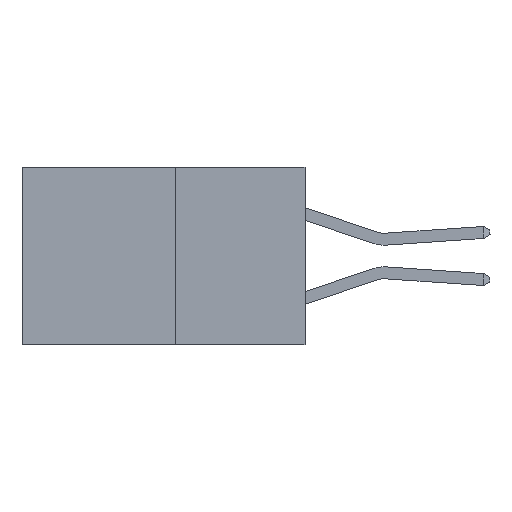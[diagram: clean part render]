
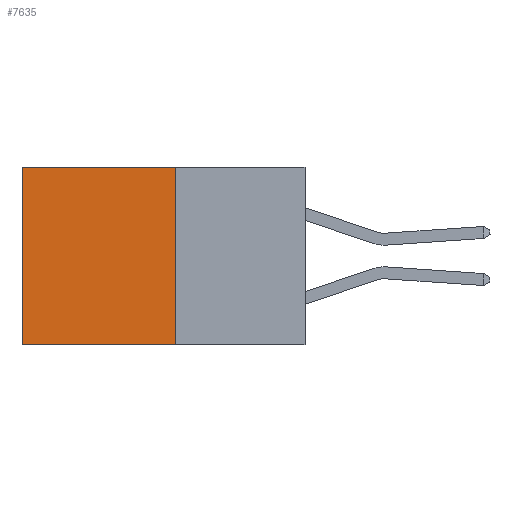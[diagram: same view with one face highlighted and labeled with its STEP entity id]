
A CAD part, left-side view. The second image highlights one B-rep face of the part: STEP entity #7635.
In plain terms, the highlighted planar face has unit normal (-1, 0, 0).
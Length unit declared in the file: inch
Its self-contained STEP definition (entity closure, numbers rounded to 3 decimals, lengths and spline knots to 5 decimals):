
#502 = VECTOR ( 'NONE', #4744, 39.37008 ) ;
#523 = LINE ( 'NONE', #7205, #9008 ) ;
#785 = VECTOR ( 'NONE', #6445, 39.37008 ) ;
#929 = VECTOR ( 'NONE', #1100, 39.37008 ) ;
#1100 = DIRECTION ( 'NONE',  ( 0., 1., 0. ) ) ;
#2003 = EDGE_CURVE ( 'NONE', #2526, #7142, #4891, .T. ) ;
#2526 = VERTEX_POINT ( 'NONE', #4250 ) ;
#2650 = LINE ( 'NONE', #2837, #502 ) ;
#2782 = VERTEX_POINT ( 'NONE', #6584 ) ;
#2837 = CARTESIAN_POINT ( 'NONE',  ( 0.277, 0.27, -0.37 ) ) ;
#4250 = CARTESIAN_POINT ( 'NONE',  ( 0.277, 0.27, 0. ) ) ;
#4744 = DIRECTION ( 'NONE',  ( 0., 1., 0. ) ) ;
#4891 = LINE ( 'NONE', #8728, #785 ) ;
#5030 = CARTESIAN_POINT ( 'NONE',  ( 0.277, 0.59, -0.37 ) ) ;
#5105 = EDGE_CURVE ( 'NONE', #2526, #2782, #5284, .T. ) ;
#5284 = LINE ( 'NONE', #9351, #929 ) ;
#5449 = ORIENTED_EDGE ( 'NONE', *, *, #6275, .T. ) ;
#6275 = EDGE_CURVE ( 'NONE', #2782, #9321, #523, .T. ) ;
#6445 = DIRECTION ( 'NONE',  ( 0., 0., -1. ) ) ;
#6584 = CARTESIAN_POINT ( 'NONE',  ( 0.277, 0.59, 0. ) ) ;
#6620 = EDGE_LOOP ( 'NONE', ( #5449, #6915, #9534, #7563 ) ) ;
#6915 = ORIENTED_EDGE ( 'NONE', *, *, #7897, .F. ) ;
#7142 = VERTEX_POINT ( 'NONE', #7643 ) ;
#7205 = CARTESIAN_POINT ( 'NONE',  ( 0.277, 0.59, -0.37 ) ) ;
#7265 = DIRECTION ( 'NONE',  ( 0., 0., -1. ) ) ;
#7563 = ORIENTED_EDGE ( 'NONE', *, *, #5105, .T. ) ;
#7635 = ADVANCED_FACE ( 'NONE', ( #9346 ), #8468, .F. ) ;
#7643 = CARTESIAN_POINT ( 'NONE',  ( 0.277, 0.27, -0.37 ) ) ;
#7709 = DIRECTION ( 'NONE',  ( 0., 0., -1. ) ) ;
#7897 = EDGE_CURVE ( 'NONE', #7142, #9321, #2650, .T. ) ;
#8468 = PLANE ( 'NONE',  #8765 ) ;
#8652 = CARTESIAN_POINT ( 'NONE',  ( 0.277, 0.27, -0.37 ) ) ;
#8728 = CARTESIAN_POINT ( 'NONE',  ( 0.277, 0.27, -0.37 ) ) ;
#8765 = AXIS2_PLACEMENT_3D ( 'NONE', #8652, #10031, #7709 ) ;
#9008 = VECTOR ( 'NONE', #7265, 39.37008 ) ;
#9321 = VERTEX_POINT ( 'NONE', #5030 ) ;
#9346 = FACE_OUTER_BOUND ( 'NONE', #6620, .T. ) ;
#9351 = CARTESIAN_POINT ( 'NONE',  ( 0.277, 0.27, 0. ) ) ;
#9534 = ORIENTED_EDGE ( 'NONE', *, *, #2003, .F. ) ;
#10031 = DIRECTION ( 'NONE',  ( 1., 0., 0. ) ) ;
